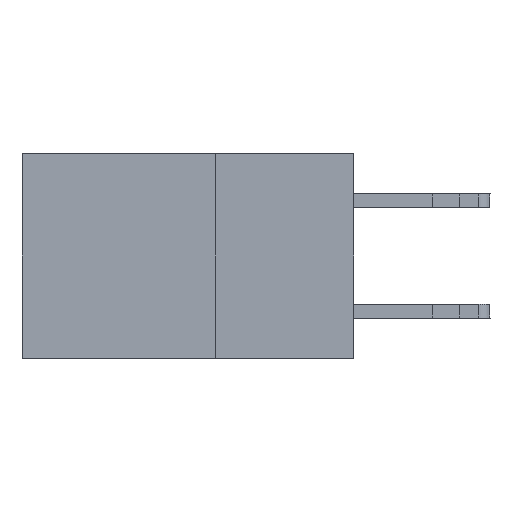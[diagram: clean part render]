
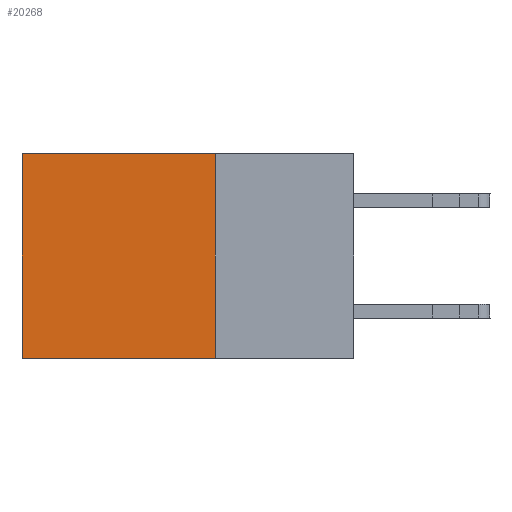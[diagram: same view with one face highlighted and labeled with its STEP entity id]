
A CAD part, left-side view. The second image highlights one B-rep face of the part: STEP entity #20268.
In plain terms, the highlighted planar face has unit normal (-1, 0, 0).
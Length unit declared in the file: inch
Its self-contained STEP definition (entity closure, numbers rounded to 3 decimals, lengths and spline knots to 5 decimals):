
#109 = LINE ( 'NONE', #475, #260 ) ;
#260 = VECTOR ( 'NONE', #12989, 39.37008 ) ;
#475 = CARTESIAN_POINT ( 'NONE',  ( 0.2875, 0.25, 0. ) ) ;
#1631 = CARTESIAN_POINT ( 'NONE',  ( 0.2875, 0.6, 0. ) ) ;
#2151 = ORIENTED_EDGE ( 'NONE', *, *, #11737, .T. ) ;
#2864 = CARTESIAN_POINT ( 'NONE',  ( 0.2875, 0.25, 0. ) ) ;
#3388 = EDGE_CURVE ( 'NONE', #6293, #9240, #109, .T. ) ;
#4567 = CARTESIAN_POINT ( 'NONE',  ( 0.2875, 0.25, 0. ) ) ;
#4965 = LINE ( 'NONE', #17727, #17947 ) ;
#5006 = ORIENTED_EDGE ( 'NONE', *, *, #20678, .T. ) ;
#6072 = VERTEX_POINT ( 'NONE', #8775 ) ;
#6293 = VERTEX_POINT ( 'NONE', #2864 ) ;
#8057 = PLANE ( 'NONE',  #14666 ) ;
#8516 = DIRECTION ( 'NONE',  ( 0., 1., 0. ) ) ;
#8775 = CARTESIAN_POINT ( 'NONE',  ( 0.2875, 0.6, -0.37 ) ) ;
#9240 = VERTEX_POINT ( 'NONE', #10882 ) ;
#10067 = CARTESIAN_POINT ( 'NONE',  ( 0.2875, 0.25, 0. ) ) ;
#10289 = LINE ( 'NONE', #4567, #18104 ) ;
#10882 = CARTESIAN_POINT ( 'NONE',  ( 0.2875, 0.25, -0.37 ) ) ;
#11166 = LINE ( 'NONE', #15210, #18465 ) ;
#11737 = EDGE_CURVE ( 'NONE', #16035, #6072, #4965, .T. ) ;
#12989 = DIRECTION ( 'NONE',  ( 0., 0., -1. ) ) ;
#12999 = EDGE_LOOP ( 'NONE', ( #2151, #22746, #22891, #5006 ) ) ;
#14666 = AXIS2_PLACEMENT_3D ( 'NONE', #10067, #17355, #15682 ) ;
#15210 = CARTESIAN_POINT ( 'NONE',  ( 0.2875, 0.25, -0.37 ) ) ;
#15682 = DIRECTION ( 'NONE',  ( 0., 0., -1. ) ) ;
#15803 = FACE_OUTER_BOUND ( 'NONE', #12999, .T. ) ;
#16035 = VERTEX_POINT ( 'NONE', #1631 ) ;
#17355 = DIRECTION ( 'NONE',  ( 1., 0., 0. ) ) ;
#17727 = CARTESIAN_POINT ( 'NONE',  ( 0.2875, 0.6, 0. ) ) ;
#17947 = VECTOR ( 'NONE', #23453, 39.37008 ) ;
#18104 = VECTOR ( 'NONE', #8516, 39.37008 ) ;
#18465 = VECTOR ( 'NONE', #18895, 39.37008 ) ;
#18895 = DIRECTION ( 'NONE',  ( 0., 1., 0. ) ) ;
#20150 = EDGE_CURVE ( 'NONE', #9240, #6072, #11166, .T. ) ;
#20268 = ADVANCED_FACE ( 'NONE', ( #15803 ), #8057, .F. ) ;
#20678 = EDGE_CURVE ( 'NONE', #6293, #16035, #10289, .T. ) ;
#22746 = ORIENTED_EDGE ( 'NONE', *, *, #20150, .F. ) ;
#22891 = ORIENTED_EDGE ( 'NONE', *, *, #3388, .F. ) ;
#23453 = DIRECTION ( 'NONE',  ( 0., 0., -1. ) ) ;
